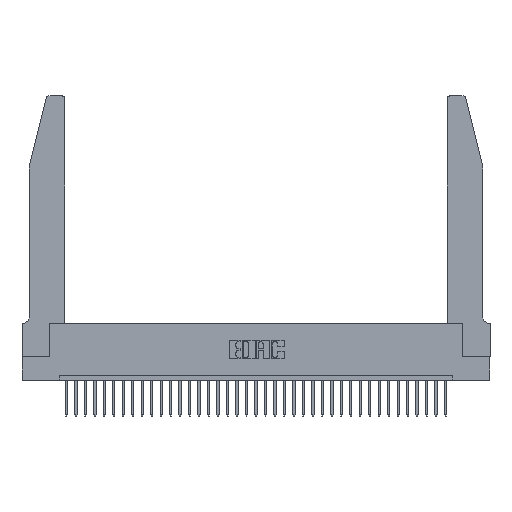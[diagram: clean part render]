
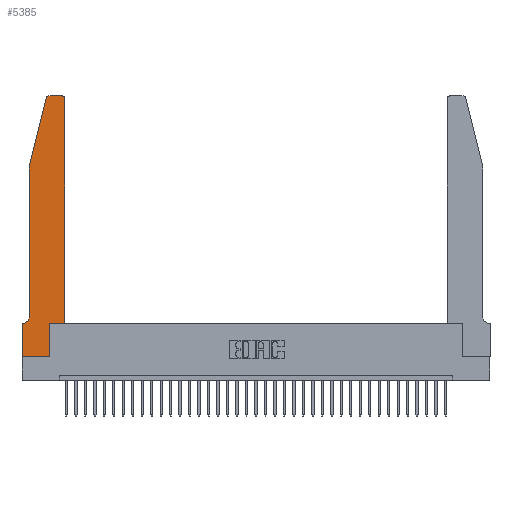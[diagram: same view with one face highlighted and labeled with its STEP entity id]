
A CAD part, top view. The second image highlights one B-rep face of the part: STEP entity #5385.
In plain terms, the highlighted planar face has unit normal (0, 0, 1).
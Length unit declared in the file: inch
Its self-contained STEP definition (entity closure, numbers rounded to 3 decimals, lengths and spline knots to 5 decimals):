
#497 = PLANE ( 'NONE',  #20066 ) ;
#725 = CARTESIAN_POINT ( 'NONE',  ( 0.25487, 2.72718, 0.37 ) ) ;
#1453 = ORIENTED_EDGE ( 'NONE', *, *, #6884, .T. ) ;
#2206 = CARTESIAN_POINT ( 'NONE',  ( 0., 0., 0.37 ) ) ;
#2546 = CARTESIAN_POINT ( 'NONE',  ( 0., 0.35, 0.37 ) ) ;
#4326 = CARTESIAN_POINT ( 'NONE',  ( 0.4205, 2.75, 0.37 ) ) ;
#4577 = VERTEX_POINT ( 'NONE', #32827 ) ;
#4609 = DIRECTION ( 'NONE',  ( 0., 0., -1. ) ) ;
#4618 = VECTOR ( 'NONE', #6152, 39.37008 ) ;
#5100 = DIRECTION ( 'NONE',  ( 0., 0., 1. ) ) ;
#5297 = AXIS2_PLACEMENT_3D ( 'NONE', #23862, #4609, #7279 ) ;
#5385 = ADVANCED_FACE ( 'NONE', ( #25113 ), #497, .T. ) ;
#5470 = LINE ( 'NONE', #14974, #4618 ) ;
#5811 = ORIENTED_EDGE ( 'NONE', *, *, #26194, .T. ) ;
#6152 = DIRECTION ( 'NONE',  ( -0.239, -0.971, 0. ) ) ;
#6278 = VECTOR ( 'NONE', #32763, 39.37008 ) ;
#6430 = VECTOR ( 'NONE', #9080, 39.37008 ) ;
#6495 = VERTEX_POINT ( 'NONE', #26849 ) ;
#6884 = EDGE_CURVE ( 'NONE', #11870, #32572, #23371, .T. ) ;
#6904 = LINE ( 'NONE', #24192, #21237 ) ;
#7050 = EDGE_CURVE ( 'NONE', #26403, #9183, #6904, .T. ) ;
#7279 = DIRECTION ( 'NONE',  ( -1., 0., 0. ) ) ;
#7641 = DIRECTION ( 'NONE',  ( 0., 1., 0. ) ) ;
#8518 = DIRECTION ( 'NONE',  ( 0., 0., 1. ) ) ;
#8558 = EDGE_CURVE ( 'NONE', #33749, #12232, #5470, .T. ) ;
#9080 = DIRECTION ( 'NONE',  ( 1., 0., 0. ) ) ;
#9183 = VERTEX_POINT ( 'NONE', #34686 ) ;
#9255 = VECTOR ( 'NONE', #18851, 39.37008 ) ;
#9452 = VERTEX_POINT ( 'NONE', #2546 ) ;
#9553 = EDGE_CURVE ( 'NONE', #9183, #23035, #32642, .T. ) ;
#10299 = AXIS2_PLACEMENT_3D ( 'NONE', #13509, #8518, #27802 ) ;
#10330 = DIRECTION ( 'NONE',  ( 1., 0., 0. ) ) ;
#10668 = DIRECTION ( 'NONE',  ( 1., 0., 0. ) ) ;
#10802 = ORIENTED_EDGE ( 'NONE', *, *, #11356, .T. ) ;
#11014 = DIRECTION ( 'NONE',  ( 0., -1., 0. ) ) ;
#11355 = EDGE_LOOP ( 'NONE', ( #15235, #10802, #11693, #5811, #31737, #19901, #26230, #1453, #23771, #32857, #14261, #14599 ) ) ;
#11356 = EDGE_CURVE ( 'NONE', #17175, #33749, #26038, .T. ) ;
#11693 = ORIENTED_EDGE ( 'NONE', *, *, #8558, .T. ) ;
#11870 = VERTEX_POINT ( 'NONE', #14398 ) ;
#11935 = EDGE_CURVE ( 'NONE', #23035, #17175, #32083, .T. ) ;
#12232 = VERTEX_POINT ( 'NONE', #14632 ) ;
#13235 = EDGE_CURVE ( 'NONE', #32629, #26403, #13808, .T. ) ;
#13509 = CARTESIAN_POINT ( 'NONE',  ( 0.284, 2.72, 0.37 ) ) ;
#13808 = LINE ( 'NONE', #25265, #6430 ) ;
#14261 = ORIENTED_EDGE ( 'NONE', *, *, #7050, .T. ) ;
#14398 = CARTESIAN_POINT ( 'NONE',  ( 0., 0., 0.37 ) ) ;
#14599 = ORIENTED_EDGE ( 'NONE', *, *, #9553, .T. ) ;
#14632 = CARTESIAN_POINT ( 'NONE',  ( 0.0755, 2., 0.37 ) ) ;
#14708 = CIRCLE ( 'NONE', #5297, 0.07 ) ;
#14891 = LINE ( 'NONE', #29829, #9255 ) ;
#14974 = CARTESIAN_POINT ( 'NONE',  ( 0.0755, 2., 0.37 ) ) ;
#15235 = ORIENTED_EDGE ( 'NONE', *, *, #11935, .T. ) ;
#17157 = CARTESIAN_POINT ( 'NONE',  ( 0.284, 2.75, 0.37 ) ) ;
#17175 = VERTEX_POINT ( 'NONE', #17157 ) ;
#17377 = VECTOR ( 'NONE', #31049, 39.37008 ) ;
#18137 = DIRECTION ( 'NONE',  ( 0., 0., 1. ) ) ;
#18774 = DIRECTION ( 'NONE',  ( 0., -1., 0. ) ) ;
#18810 = CARTESIAN_POINT ( 'NONE',  ( 0., 0.35, 0.37 ) ) ;
#18851 = DIRECTION ( 'NONE',  ( 0., 1., 0. ) ) ;
#19270 = CARTESIAN_POINT ( 'NONE',  ( 0., 0., 0.37 ) ) ;
#19800 = CARTESIAN_POINT ( 'NONE',  ( 0.4505, 0.35, 0.37 ) ) ;
#19901 = ORIENTED_EDGE ( 'NONE', *, *, #21479, .T. ) ;
#20055 = VECTOR ( 'NONE', #18774, 39.37008 ) ;
#20066 = AXIS2_PLACEMENT_3D ( 'NONE', #18810, #5100, #10668 ) ;
#20904 = DIRECTION ( 'NONE',  ( 1., 0., 0. ) ) ;
#21237 = VECTOR ( 'NONE', #7641, 39.37008 ) ;
#21479 = EDGE_CURVE ( 'NONE', #4577, #9452, #30953, .T. ) ;
#21639 = VECTOR ( 'NONE', #10330, 39.37008 ) ;
#23035 = VERTEX_POINT ( 'NONE', #4326 ) ;
#23290 = EDGE_CURVE ( 'NONE', #32572, #32629, #14891, .T. ) ;
#23371 = LINE ( 'NONE', #2206, #21639 ) ;
#23579 = VECTOR ( 'NONE', #11014, 39.37008 ) ;
#23771 = ORIENTED_EDGE ( 'NONE', *, *, #23290, .T. ) ;
#23862 = CARTESIAN_POINT ( 'NONE',  ( 0.0055, 0.42, 0.37 ) ) ;
#24192 = CARTESIAN_POINT ( 'NONE',  ( 0.4505, 0.35, 0.37 ) ) ;
#24633 = CARTESIAN_POINT ( 'NONE',  ( 0.0755, 2., 0.37 ) ) ;
#25113 = FACE_OUTER_BOUND ( 'NONE', #11355, .T. ) ;
#25265 = CARTESIAN_POINT ( 'NONE',  ( 0.4505, 0.35, 0.37 ) ) ;
#25597 = EDGE_CURVE ( 'NONE', #9452, #11870, #28764, .T. ) ;
#26038 = CIRCLE ( 'NONE', #10299, 0.03 ) ;
#26194 = EDGE_CURVE ( 'NONE', #12232, #6495, #30425, .T. ) ;
#26230 = ORIENTED_EDGE ( 'NONE', *, *, #25597, .T. ) ;
#26403 = VERTEX_POINT ( 'NONE', #19800 ) ;
#26849 = CARTESIAN_POINT ( 'NONE',  ( 0.0755, 0.42, 0.37 ) ) ;
#27605 = CARTESIAN_POINT ( 'NONE',  ( 0.0755, 0.35, 0.37 ) ) ;
#27802 = DIRECTION ( 'NONE',  ( 1., 0., 0. ) ) ;
#28108 = EDGE_CURVE ( 'NONE', #6495, #4577, #14708, .T. ) ;
#28764 = LINE ( 'NONE', #19270, #23579 ) ;
#29676 = AXIS2_PLACEMENT_3D ( 'NONE', #31862, #18137, #20904 ) ;
#29829 = CARTESIAN_POINT ( 'NONE',  ( 0.2865, 0.35, 0.37 ) ) ;
#29842 = CARTESIAN_POINT ( 'NONE',  ( 0.2865, 0.35, 0.37 ) ) ;
#30425 = LINE ( 'NONE', #24633, #20055 ) ;
#30953 = LINE ( 'NONE', #27605, #6278 ) ;
#31049 = DIRECTION ( 'NONE',  ( -1., 0., 0. ) ) ;
#31291 = CARTESIAN_POINT ( 'NONE',  ( 0.2605, 2.75, 0.37 ) ) ;
#31737 = ORIENTED_EDGE ( 'NONE', *, *, #28108, .T. ) ;
#31862 = CARTESIAN_POINT ( 'NONE',  ( 0.4205, 2.72, 0.37 ) ) ;
#32083 = LINE ( 'NONE', #31291, #17377 ) ;
#32572 = VERTEX_POINT ( 'NONE', #32709 ) ;
#32629 = VERTEX_POINT ( 'NONE', #29842 ) ;
#32642 = CIRCLE ( 'NONE', #29676, 0.03 ) ;
#32709 = CARTESIAN_POINT ( 'NONE',  ( 0.2865, 0., 0.37 ) ) ;
#32763 = DIRECTION ( 'NONE',  ( -1., 0., 0. ) ) ;
#32827 = CARTESIAN_POINT ( 'NONE',  ( 0.0055, 0.35, 0.37 ) ) ;
#32857 = ORIENTED_EDGE ( 'NONE', *, *, #13235, .T. ) ;
#33749 = VERTEX_POINT ( 'NONE', #725 ) ;
#34686 = CARTESIAN_POINT ( 'NONE',  ( 0.4505, 2.72, 0.37 ) ) ;
